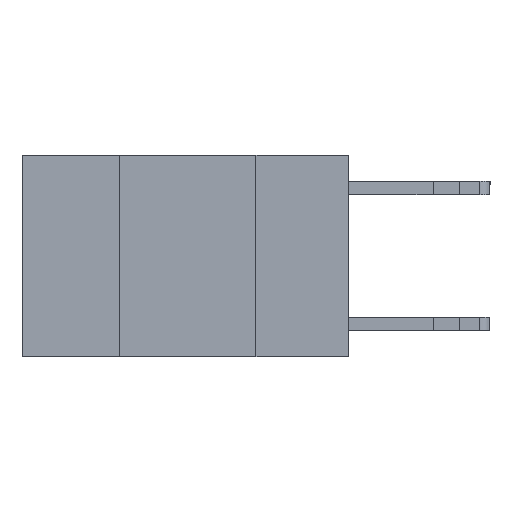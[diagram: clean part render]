
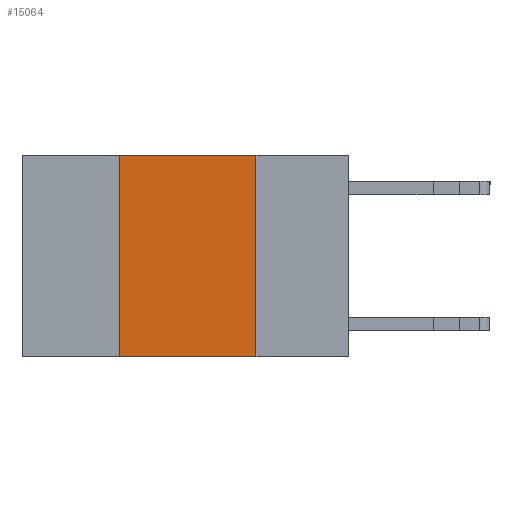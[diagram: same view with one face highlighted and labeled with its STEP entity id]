
A CAD part, left-side view. The second image highlights one B-rep face of the part: STEP entity #15064.
In plain terms, the highlighted planar face has unit normal (-1, 0, 0).
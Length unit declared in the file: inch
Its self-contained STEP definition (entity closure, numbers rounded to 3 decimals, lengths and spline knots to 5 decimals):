
#1411 = DIRECTION ( 'NONE',  ( 1., 0., 0. ) ) ;
#1758 = CARTESIAN_POINT ( 'NONE',  ( 0., 0.17, 0. ) ) ;
#1813 = VECTOR ( 'NONE', #3641, 39.37008 ) ;
#2496 = DIRECTION ( 'NONE',  ( 0., -1., 0. ) ) ;
#2598 = EDGE_LOOP ( 'NONE', ( #3880, #8270, #3157, #12144 ) ) ;
#2713 = VECTOR ( 'NONE', #12272, 39.37008 ) ;
#2770 = EDGE_CURVE ( 'NONE', #12014, #15782, #5218, .T. ) ;
#3157 = ORIENTED_EDGE ( 'NONE', *, *, #10672, .F. ) ;
#3641 = DIRECTION ( 'NONE',  ( 0., -1., 0. ) ) ;
#3752 = CARTESIAN_POINT ( 'NONE',  ( 0., 0.6, 0. ) ) ;
#3789 = VECTOR ( 'NONE', #2496, 39.37008 ) ;
#3880 = ORIENTED_EDGE ( 'NONE', *, *, #2770, .F. ) ;
#4268 = CARTESIAN_POINT ( 'NONE',  ( 0., 0.17, 0. ) ) ;
#4417 = VECTOR ( 'NONE', #15000, 39.37008 ) ;
#5218 = LINE ( 'NONE', #1758, #2713 ) ;
#5631 = VERTEX_POINT ( 'NONE', #15368 ) ;
#7121 = EDGE_CURVE ( 'NONE', #14369, #15782, #9947, .T. ) ;
#8270 = ORIENTED_EDGE ( 'NONE', *, *, #13611, .F. ) ;
#8298 = CARTESIAN_POINT ( 'NONE',  ( 0., 0.17, -0.37 ) ) ;
#9455 = CARTESIAN_POINT ( 'NONE',  ( 0., 0.42, -0.37 ) ) ;
#9947 = LINE ( 'NONE', #11304, #1813 ) ;
#10063 = LINE ( 'NONE', #12498, #4417 ) ;
#10672 = EDGE_CURVE ( 'NONE', #14369, #5631, #10063, .T. ) ;
#11304 = CARTESIAN_POINT ( 'NONE',  ( 0., 0.6, -0.37 ) ) ;
#12014 = VERTEX_POINT ( 'NONE', #4268 ) ;
#12144 = ORIENTED_EDGE ( 'NONE', *, *, #7121, .T. ) ;
#12272 = DIRECTION ( 'NONE',  ( 0., 0., -1. ) ) ;
#12416 = AXIS2_PLACEMENT_3D ( 'NONE', #14361, #1411, #12850 ) ;
#12420 = LINE ( 'NONE', #3752, #3789 ) ;
#12436 = FACE_OUTER_BOUND ( 'NONE', #2598, .T. ) ;
#12498 = CARTESIAN_POINT ( 'NONE',  ( 0., 0.42, 0. ) ) ;
#12686 = PLANE ( 'NONE',  #12416 ) ;
#12850 = DIRECTION ( 'NONE',  ( 0., 0., -1. ) ) ;
#13611 = EDGE_CURVE ( 'NONE', #5631, #12014, #12420, .T. ) ;
#14361 = CARTESIAN_POINT ( 'NONE',  ( 0., 0.6, 0. ) ) ;
#14369 = VERTEX_POINT ( 'NONE', #9455 ) ;
#15000 = DIRECTION ( 'NONE',  ( 0., 0., 1. ) ) ;
#15064 = ADVANCED_FACE ( 'NONE', ( #12436 ), #12686, .F. ) ;
#15368 = CARTESIAN_POINT ( 'NONE',  ( 0., 0.42, 0. ) ) ;
#15782 = VERTEX_POINT ( 'NONE', #8298 ) ;
